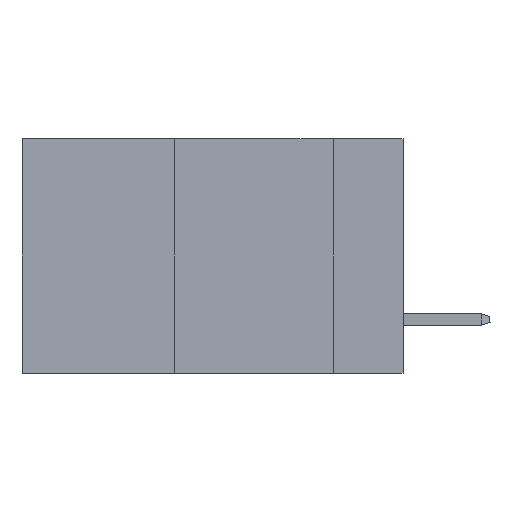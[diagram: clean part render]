
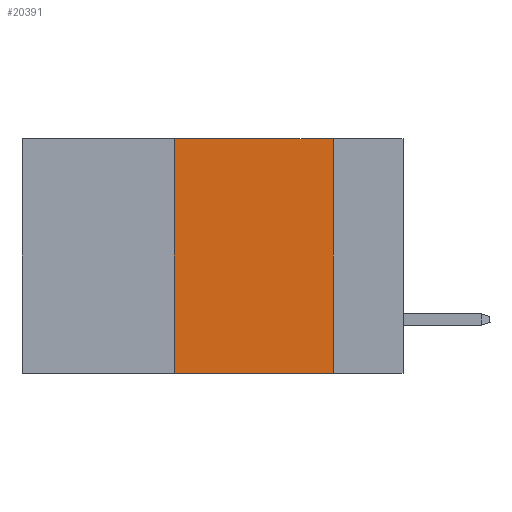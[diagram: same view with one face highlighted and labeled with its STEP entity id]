
A CAD part, left-side view. The second image highlights one B-rep face of the part: STEP entity #20391.
In plain terms, the highlighted planar face has unit normal (-1, 0, 0).
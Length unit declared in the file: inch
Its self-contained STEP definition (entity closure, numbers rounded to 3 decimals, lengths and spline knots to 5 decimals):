
#542 = CARTESIAN_POINT ( 'NONE',  ( 0., 0.36, 0. ) ) ;
#2388 = LINE ( 'NONE', #2520, #12172 ) ;
#2520 = CARTESIAN_POINT ( 'NONE',  ( 0., 0.11, 0. ) ) ;
#2674 = CARTESIAN_POINT ( 'NONE',  ( 0., 0.6, 0. ) ) ;
#3600 = AXIS2_PLACEMENT_3D ( 'NONE', #24980, #6827, #22336 ) ;
#6690 = PLANE ( 'NONE',  #3600 ) ;
#6827 = DIRECTION ( 'NONE',  ( 1., 0., 0. ) ) ;
#7067 = ORIENTED_EDGE ( 'NONE', *, *, #16192, .T. ) ;
#8570 = EDGE_CURVE ( 'NONE', #21859, #12984, #2388, .T. ) ;
#9134 = VERTEX_POINT ( 'NONE', #16084 ) ;
#9210 = ORIENTED_EDGE ( 'NONE', *, *, #21966, .F. ) ;
#9655 = EDGE_CURVE ( 'NONE', #15921, #9134, #16578, .T. ) ;
#10785 = LINE ( 'NONE', #12508, #25122 ) ;
#12172 = VECTOR ( 'NONE', #18548, 39.37008 ) ;
#12192 = ORIENTED_EDGE ( 'NONE', *, *, #9655, .F. ) ;
#12508 = CARTESIAN_POINT ( 'NONE',  ( 0., 0.6, -0.37 ) ) ;
#12741 = DIRECTION ( 'NONE',  ( 0., 0., 1. ) ) ;
#12984 = VERTEX_POINT ( 'NONE', #24868 ) ;
#13070 = VECTOR ( 'NONE', #12741, 39.37008 ) ;
#13630 = ORIENTED_EDGE ( 'NONE', *, *, #8570, .F. ) ;
#14631 = LINE ( 'NONE', #2674, #18187 ) ;
#15475 = CARTESIAN_POINT ( 'NONE',  ( 0., 0.11, 0. ) ) ;
#15565 = CARTESIAN_POINT ( 'NONE',  ( 0., 0.36, -0.37 ) ) ;
#15921 = VERTEX_POINT ( 'NONE', #15565 ) ;
#16084 = CARTESIAN_POINT ( 'NONE',  ( 0., 0.36, 0. ) ) ;
#16192 = EDGE_CURVE ( 'NONE', #15921, #12984, #10785, .T. ) ;
#16578 = LINE ( 'NONE', #542, #13070 ) ;
#17006 = DIRECTION ( 'NONE',  ( 0., -1., 0. ) ) ;
#18187 = VECTOR ( 'NONE', #18841, 39.37008 ) ;
#18548 = DIRECTION ( 'NONE',  ( 0., 0., -1. ) ) ;
#18841 = DIRECTION ( 'NONE',  ( 0., -1., 0. ) ) ;
#19329 = EDGE_LOOP ( 'NONE', ( #13630, #9210, #12192, #7067 ) ) ;
#20391 = ADVANCED_FACE ( 'NONE', ( #24860 ), #6690, .F. ) ;
#21859 = VERTEX_POINT ( 'NONE', #15475 ) ;
#21966 = EDGE_CURVE ( 'NONE', #9134, #21859, #14631, .T. ) ;
#22336 = DIRECTION ( 'NONE',  ( 0., 0., -1. ) ) ;
#24860 = FACE_OUTER_BOUND ( 'NONE', #19329, .T. ) ;
#24868 = CARTESIAN_POINT ( 'NONE',  ( 0., 0.11, -0.37 ) ) ;
#24980 = CARTESIAN_POINT ( 'NONE',  ( 0., 0.6, 0. ) ) ;
#25122 = VECTOR ( 'NONE', #17006, 39.37008 ) ;
